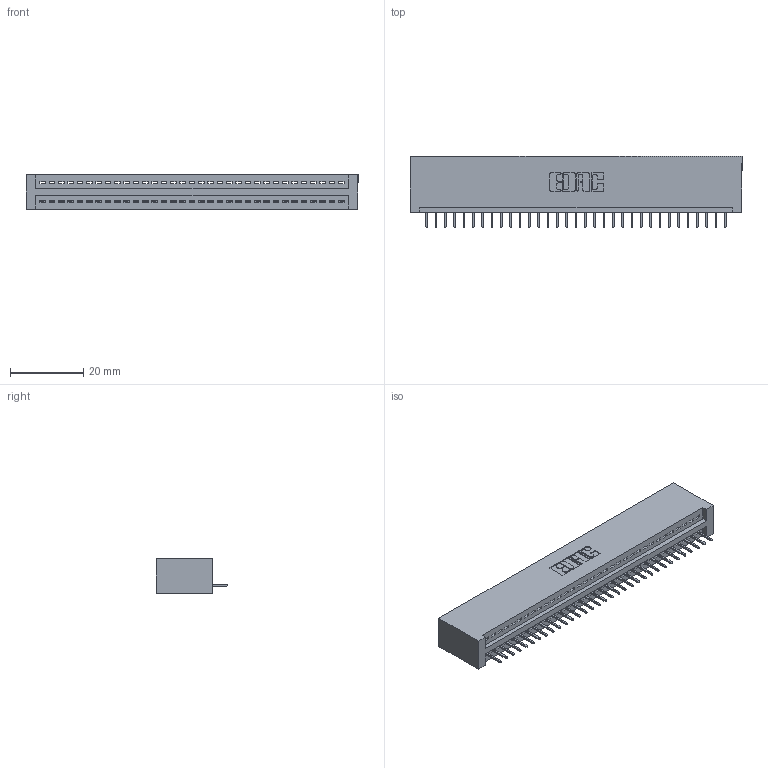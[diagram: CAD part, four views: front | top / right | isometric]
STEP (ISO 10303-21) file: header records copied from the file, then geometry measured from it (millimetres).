
FILE_DESCRIPTION (( 'STEP AP203' ), '1' );
FILE_NAME ('345-033-524-101.STEP', '2019-10-07T15:55:53', ( '' ), ( '' ), 'SwSTEP 2.0', 'SolidWorks 2016', '' );
FILE_SCHEMA (( 'CONFIG_CONTROL_DESIGN' ));
Length unit declared in the file: inch
Products named in the file (3): 345-292-001_345-293-124; 345 Part_No Mounting Lugs; 345-033-524-101
Assembly tree (34 placements, depth 2):
  345-033-524-101
    345 Part_No Mounting Lugs
    345-292-001_345-293-124  x33
Bounding box: 90.42 x 19.35 x 9.4 mm (x, y, z)
Volume: 8968.8 mm3; surface area: 11569.8 mm2
Topology: 34 solids, 34 shells, 2164 faces, 6257 edges, 4038 vertices
Faces by surface type: plane 1594, cylinder 570
Entity records: 25845 total; most frequent: CARTESIAN_POINT 4483, ORIENTED_EDGE 4450, DIRECTION 3923, EDGE_CURVE 2225, LINE 1973, VECTOR 1973, VERTEX_POINT 1478, AXIS2_PLACEMENT_3D 975
